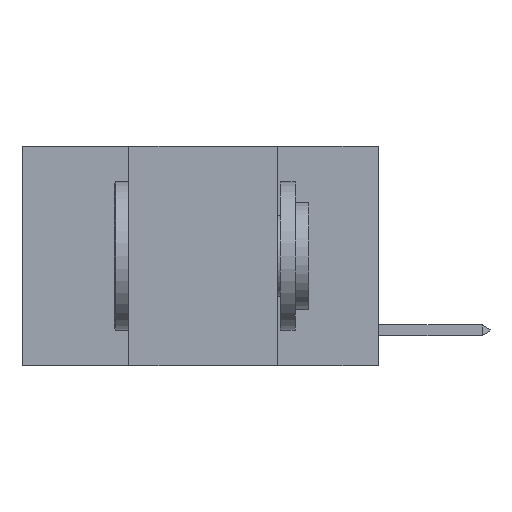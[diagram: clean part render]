
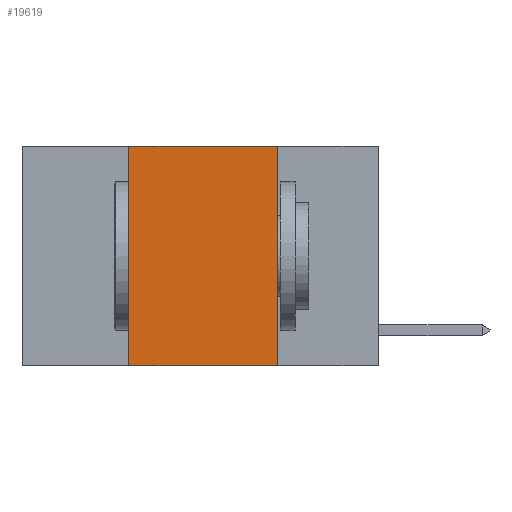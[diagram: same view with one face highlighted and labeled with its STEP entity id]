
A CAD part, left-side view. The second image highlights one B-rep face of the part: STEP entity #19619.
In plain terms, the highlighted planar face has unit normal (-1, 0, 0).
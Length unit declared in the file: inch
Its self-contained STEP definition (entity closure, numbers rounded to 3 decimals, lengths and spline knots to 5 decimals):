
#495 = DIRECTION ( 'NONE',  ( 1., 0., 0. ) ) ;
#1666 = VERTEX_POINT ( 'NONE', #19132 ) ;
#1705 = LINE ( 'NONE', #4078, #23853 ) ;
#2297 = VECTOR ( 'NONE', #17069, 39.37008 ) ;
#2739 = LINE ( 'NONE', #17740, #26945 ) ;
#4078 = CARTESIAN_POINT ( 'NONE',  ( 0., 0.42, 0. ) ) ;
#5636 = CARTESIAN_POINT ( 'NONE',  ( 0., 0.42, 0. ) ) ;
#6662 = CARTESIAN_POINT ( 'NONE',  ( 0., 0.6, 0. ) ) ;
#7764 = CARTESIAN_POINT ( 'NONE',  ( 0., 0.17, 0. ) ) ;
#7765 = EDGE_CURVE ( 'NONE', #18131, #1666, #12800, .T. ) ;
#8386 = CARTESIAN_POINT ( 'NONE',  ( 0., 0.6, 0. ) ) ;
#11869 = ORIENTED_EDGE ( 'NONE', *, *, #25097, .T. ) ;
#12800 = LINE ( 'NONE', #8386, #2297 ) ;
#13909 = CARTESIAN_POINT ( 'NONE',  ( 0., 0.42, -0.37 ) ) ;
#14867 = VERTEX_POINT ( 'NONE', #13909 ) ;
#15549 = AXIS2_PLACEMENT_3D ( 'NONE', #6662, #495, #19444 ) ;
#16418 = DIRECTION ( 'NONE',  ( 0., 0., -1. ) ) ;
#17069 = DIRECTION ( 'NONE',  ( 0., -1., 0. ) ) ;
#17740 = CARTESIAN_POINT ( 'NONE',  ( 0., 0.6, -0.37 ) ) ;
#18131 = VERTEX_POINT ( 'NONE', #5636 ) ;
#18134 = EDGE_CURVE ( 'NONE', #1666, #23842, #18707, .T. ) ;
#18707 = LINE ( 'NONE', #7764, #24072 ) ;
#19132 = CARTESIAN_POINT ( 'NONE',  ( 0., 0.17, 0. ) ) ;
#19444 = DIRECTION ( 'NONE',  ( 0., 0., -1. ) ) ;
#19602 = DIRECTION ( 'NONE',  ( 0., -1., 0. ) ) ;
#19619 = ADVANCED_FACE ( 'NONE', ( #21995 ), #19861, .F. ) ;
#19861 = PLANE ( 'NONE',  #15549 ) ;
#21840 = ORIENTED_EDGE ( 'NONE', *, *, #18134, .F. ) ;
#21995 = FACE_OUTER_BOUND ( 'NONE', #25200, .T. ) ;
#23077 = DIRECTION ( 'NONE',  ( 0., 0., 1. ) ) ;
#23842 = VERTEX_POINT ( 'NONE', #26508 ) ;
#23853 = VECTOR ( 'NONE', #23077, 39.37008 ) ;
#24072 = VECTOR ( 'NONE', #16418, 39.37008 ) ;
#24198 = ORIENTED_EDGE ( 'NONE', *, *, #7765, .F. ) ;
#25097 = EDGE_CURVE ( 'NONE', #14867, #23842, #2739, .T. ) ;
#25200 = EDGE_LOOP ( 'NONE', ( #21840, #24198, #26289, #11869 ) ) ;
#25843 = EDGE_CURVE ( 'NONE', #14867, #18131, #1705, .T. ) ;
#26289 = ORIENTED_EDGE ( 'NONE', *, *, #25843, .F. ) ;
#26508 = CARTESIAN_POINT ( 'NONE',  ( 0., 0.17, -0.37 ) ) ;
#26945 = VECTOR ( 'NONE', #19602, 39.37008 ) ;
